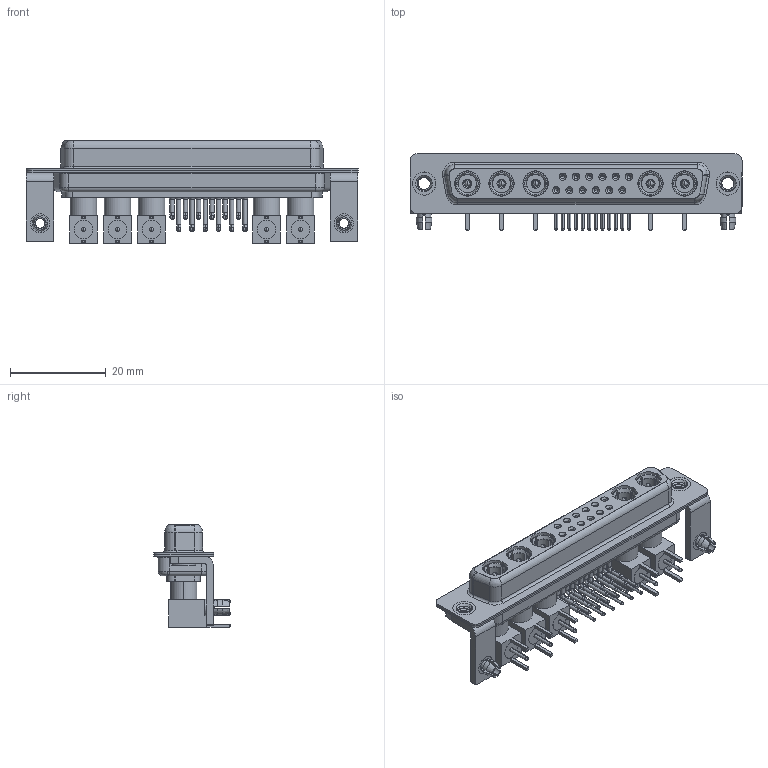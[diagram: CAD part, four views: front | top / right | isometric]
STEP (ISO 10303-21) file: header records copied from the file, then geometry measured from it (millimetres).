
FILE_DESCRIPTION (( 'STEP AP203' ), '1' );
FILE_NAME ('630-17W5240-5NB.STEP', '2022-06-06T19:15:51', ( '' ), ( '' ), 'SwSTEP 2.0', 'SolidWorks 2020', '' );
FILE_SCHEMA (( 'CONFIG_CONTROL_DESIGN' ));
Length unit declared in the file: millimetre
Products named in the file (20): 630Combo Board Lock; Locking Collar; Co-Ax Plug Assy_RA; Co-Ax Plug_RA PC Tail; Insulator RA Pin; Insulator Pin_Straight PC Tail; 630Combo Shell Front_37 Contacts; Pin_RA; 630Combo Contact Row 1; 630-17W5240-5NB; 630Combo Stabilizer Bracket; 630Combo Threaded Rivet_B; RA Back Shell; 630Combo Contact Row 2; 630Combo Housing_17W5; 630Combo Shell Rear_37 Contacts
Assembly tree (56 placements, depth 3):
  630-17W5240-5NB
    630Combo Housing_17W5
    630Combo Shell Front_37 Contacts
    630Combo Shell Rear_37 Contacts
    630Combo Threaded Rivet_B  x2
    630Combo Stabilizer Bracket  x2
    630Combo Board Lock  x2
    Co-Ax Plug Assy_RA
      Co-Ax Plug_RA PC Tail
      Insulator Pin_Straight PC Tail
      Pin_RA
      Locking Collar
      RA Back Shell
      Insulator RA Pin
    Co-Ax Plug Assy_RA
      Co-Ax Plug_RA PC Tail
      Insulator Pin_Straight PC Tail
      Pin_RA
      Locking Collar
      RA Back Shell
      Insulator RA Pin
    Co-Ax Plug Assy_RA
      Co-Ax Plug_RA PC Tail
      Insulator Pin_Straight PC Tail
      Pin_RA
      Locking Collar
      RA Back Shell
      Insulator RA Pin
    Co-Ax Plug Assy_RA
      Co-Ax Plug_RA PC Tail
      Insulator Pin_Straight PC Tail
      Pin_RA
      Locking Collar
      RA Back Shell
      Insulator RA Pin
    Co-Ax Plug Assy_RA
      Co-Ax Plug_RA PC Tail
      Insulator Pin_Straight PC Tail
      Pin_RA
      Locking Collar
      RA Back Shell
      Insulator RA Pin
    630Combo Contact Row 1  x6
    630Combo Contact Row 2  x6
Bounding box: 69.4 x 16 x 21.41 mm (x, y, z)
Volume: 6801.5 mm3; surface area: 16290 mm2
Topology: 51 solids, 51 shells, 1885 faces, 4654 edges, 2928 vertices
Faces by surface type: cylinder 788, plane 650, cone 281, torus 87, bspline 59, sphere 20
Entity records: 26736 total; most frequent: CARTESIAN_POINT 5732, DIRECTION 4097, ORIENTED_EDGE 3510, EDGE_CURVE 1755, AXIS2_PLACEMENT_3D 1674, VERTEX_POINT 1119, CIRCLE 887, EDGE_LOOP 868
